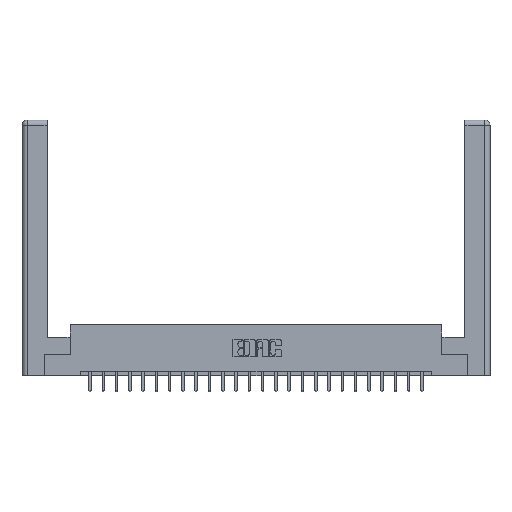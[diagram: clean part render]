
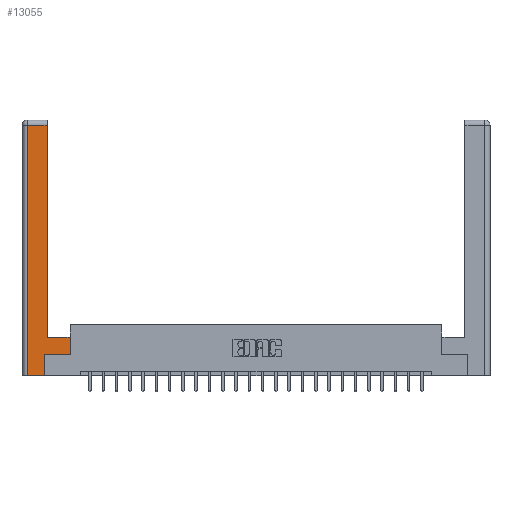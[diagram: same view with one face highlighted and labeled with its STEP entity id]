
A CAD part, top view. The second image highlights one B-rep face of the part: STEP entity #13055.
In plain terms, the highlighted planar face has unit normal (0, 0, 1).
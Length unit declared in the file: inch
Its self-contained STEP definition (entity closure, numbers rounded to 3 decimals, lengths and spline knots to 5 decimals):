
#487 = DIRECTION ( 'NONE',  ( 1., 0., 0. ) ) ;
#792 = VERTEX_POINT ( 'NONE', #1787 ) ;
#862 = EDGE_CURVE ( 'NONE', #8049, #18285, #5640, .T. ) ;
#1504 = ORIENTED_EDGE ( 'NONE', *, *, #8350, .T. ) ;
#1787 = CARTESIAN_POINT ( 'NONE',  ( 0.565, 0.245, 0. ) ) ;
#1929 = LINE ( 'NONE', #17745, #11568 ) ;
#2023 = DIRECTION ( 'NONE',  ( -1., 0., 0. ) ) ;
#2103 = EDGE_CURVE ( 'NONE', #6071, #22890, #6666, .T. ) ;
#2554 = VECTOR ( 'NONE', #15322, 39.37008 ) ;
#4188 = CARTESIAN_POINT ( 'NONE',  ( 0.295, 0.45, 0. ) ) ;
#5640 = LINE ( 'NONE', #9619, #20742 ) ;
#5841 = ORIENTED_EDGE ( 'NONE', *, *, #11746, .T. ) ;
#6071 = VERTEX_POINT ( 'NONE', #13620 ) ;
#6406 = EDGE_LOOP ( 'NONE', ( #7490, #12939, #1504, #16989, #21666, #5841, #14437, #19135 ) ) ;
#6666 = LINE ( 'NONE', #24172, #9699 ) ;
#6965 = EDGE_CURVE ( 'NONE', #18285, #6071, #1929, .T. ) ;
#7335 = CARTESIAN_POINT ( 'NONE',  ( 0.565, 0.245, 0. ) ) ;
#7490 = ORIENTED_EDGE ( 'NONE', *, *, #6965, .T. ) ;
#7702 = CARTESIAN_POINT ( 'NONE',  ( 0.265, 0.245, 0. ) ) ;
#8040 = CARTESIAN_POINT ( 'NONE',  ( 0.0615, 2.94, 0. ) ) ;
#8049 = VERTEX_POINT ( 'NONE', #21974 ) ;
#8350 = EDGE_CURVE ( 'NONE', #22890, #19858, #17823, .T. ) ;
#9443 = FACE_OUTER_BOUND ( 'NONE', #6406, .T. ) ;
#9619 = CARTESIAN_POINT ( 'NONE',  ( 0.295, 0.45, 0. ) ) ;
#9699 = VECTOR ( 'NONE', #23825, 39.37008 ) ;
#10171 = CARTESIAN_POINT ( 'NONE',  ( 0.265, 0., 0. ) ) ;
#11170 = DIRECTION ( 'NONE',  ( 0., 0., -1. ) ) ;
#11227 = AXIS2_PLACEMENT_3D ( 'NONE', #16920, #11170, #18872 ) ;
#11568 = VECTOR ( 'NONE', #13673, 39.37008 ) ;
#11746 = EDGE_CURVE ( 'NONE', #22746, #792, #19188, .T. ) ;
#11792 = VECTOR ( 'NONE', #14799, 39.37008 ) ;
#12939 = ORIENTED_EDGE ( 'NONE', *, *, #2103, .T. ) ;
#13055 = ADVANCED_FACE ( 'NONE', ( #9443 ), #16484, .F. ) ;
#13620 = CARTESIAN_POINT ( 'NONE',  ( 0.295, 2.94, 0. ) ) ;
#13673 = DIRECTION ( 'NONE',  ( 0., 1., 0. ) ) ;
#14426 = CARTESIAN_POINT ( 'NONE',  ( 0.0615, 0., 0. ) ) ;
#14437 = ORIENTED_EDGE ( 'NONE', *, *, #15019, .T. ) ;
#14799 = DIRECTION ( 'NONE',  ( 0., 1., 0. ) ) ;
#15019 = EDGE_CURVE ( 'NONE', #792, #8049, #22375, .T. ) ;
#15322 = DIRECTION ( 'NONE',  ( 1., 0., 0. ) ) ;
#15437 = CARTESIAN_POINT ( 'NONE',  ( 0.265, 0.245, 0. ) ) ;
#16484 = PLANE ( 'NONE',  #11227 ) ;
#16920 = CARTESIAN_POINT ( 'NONE',  ( 0., 0., 0. ) ) ;
#16984 = DIRECTION ( 'NONE',  ( 0., 1., 0. ) ) ;
#16989 = ORIENTED_EDGE ( 'NONE', *, *, #21587, .T. ) ;
#17745 = CARTESIAN_POINT ( 'NONE',  ( 0.295, 3., 0. ) ) ;
#17823 = LINE ( 'NONE', #14426, #22013 ) ;
#18285 = VERTEX_POINT ( 'NONE', #4188 ) ;
#18328 = CARTESIAN_POINT ( 'NONE',  ( 0.0615, 0., 0. ) ) ;
#18656 = VERTEX_POINT ( 'NONE', #22496 ) ;
#18872 = DIRECTION ( 'NONE',  ( -1., 0., 0. ) ) ;
#19135 = ORIENTED_EDGE ( 'NONE', *, *, #862, .T. ) ;
#19188 = LINE ( 'NONE', #7335, #2554 ) ;
#19485 = LINE ( 'NONE', #15437, #20374 ) ;
#19506 = EDGE_CURVE ( 'NONE', #18656, #22746, #19485, .T. ) ;
#19858 = VERTEX_POINT ( 'NONE', #18328 ) ;
#19986 = LINE ( 'NONE', #10171, #21473 ) ;
#20374 = VECTOR ( 'NONE', #16984, 39.37008 ) ;
#20742 = VECTOR ( 'NONE', #2023, 39.37008 ) ;
#21473 = VECTOR ( 'NONE', #487, 39.37008 ) ;
#21587 = EDGE_CURVE ( 'NONE', #19858, #18656, #19986, .T. ) ;
#21666 = ORIENTED_EDGE ( 'NONE', *, *, #19506, .T. ) ;
#21974 = CARTESIAN_POINT ( 'NONE',  ( 0.565, 0.45, 0. ) ) ;
#22013 = VECTOR ( 'NONE', #22015, 39.37008 ) ;
#22015 = DIRECTION ( 'NONE',  ( 0., -1., 0. ) ) ;
#22375 = LINE ( 'NONE', #22751, #11792 ) ;
#22496 = CARTESIAN_POINT ( 'NONE',  ( 0.265, 0., 0. ) ) ;
#22746 = VERTEX_POINT ( 'NONE', #7702 ) ;
#22751 = CARTESIAN_POINT ( 'NONE',  ( 0.565, 0.45, 0. ) ) ;
#22890 = VERTEX_POINT ( 'NONE', #8040 ) ;
#23825 = DIRECTION ( 'NONE',  ( -1., 0., 0. ) ) ;
#24172 = CARTESIAN_POINT ( 'NONE',  ( 0.0615, 2.94, 0. ) ) ;
